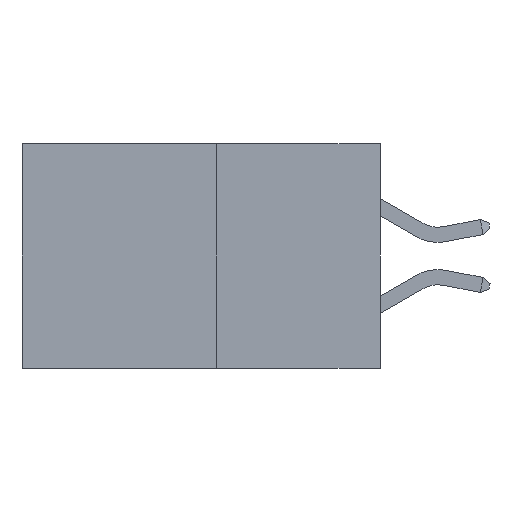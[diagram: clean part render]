
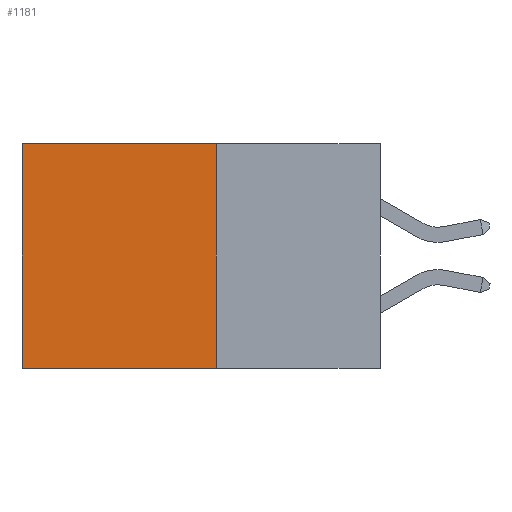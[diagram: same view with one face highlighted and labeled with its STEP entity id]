
A CAD part, left-side view. The second image highlights one B-rep face of the part: STEP entity #1181.
In plain terms, the highlighted planar face has unit normal (-1, 0, 0).
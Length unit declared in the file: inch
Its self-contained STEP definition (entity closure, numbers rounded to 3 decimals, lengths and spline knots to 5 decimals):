
#418 = CARTESIAN_POINT ( 'NONE',  ( 0.277, 0.27, 0. ) ) ;
#1023 = DIRECTION ( 'NONE',  ( 0., 0., -1. ) ) ;
#1181 = ADVANCED_FACE ( 'NONE', ( #3121 ), #8649, .F. ) ;
#1268 = CARTESIAN_POINT ( 'NONE',  ( 0.277, 0.27, -0.37 ) ) ;
#1397 = VERTEX_POINT ( 'NONE', #6415 ) ;
#1732 = DIRECTION ( 'NONE',  ( 0., 1., 0. ) ) ;
#1752 = VECTOR ( 'NONE', #1732, 39.37008 ) ;
#1997 = ORIENTED_EDGE ( 'NONE', *, *, #8250, .F. ) ;
#2171 = VERTEX_POINT ( 'NONE', #4572 ) ;
#2294 = AXIS2_PLACEMENT_3D ( 'NONE', #2335, #6677, #6979 ) ;
#2335 = CARTESIAN_POINT ( 'NONE',  ( 0.277, 0.27, -0.37 ) ) ;
#2494 = ORIENTED_EDGE ( 'NONE', *, *, #2609, .F. ) ;
#2504 = VECTOR ( 'NONE', #9385, 39.37008 ) ;
#2609 = EDGE_CURVE ( 'NONE', #1397, #2171, #6265, .T. ) ;
#2628 = EDGE_CURVE ( 'NONE', #4835, #2171, #8755, .T. ) ;
#2877 = ORIENTED_EDGE ( 'NONE', *, *, #2628, .T. ) ;
#3024 = CARTESIAN_POINT ( 'NONE',  ( 0.277, 0.59, 0. ) ) ;
#3121 = FACE_OUTER_BOUND ( 'NONE', #4414, .T. ) ;
#3892 = VECTOR ( 'NONE', #7174, 39.37008 ) ;
#3923 = EDGE_CURVE ( 'NONE', #6379, #4835, #7024, .T. ) ;
#4414 = EDGE_LOOP ( 'NONE', ( #2877, #2494, #1997, #8170 ) ) ;
#4572 = CARTESIAN_POINT ( 'NONE',  ( 0.277, 0.59, -0.37 ) ) ;
#4835 = VERTEX_POINT ( 'NONE', #3024 ) ;
#5214 = CARTESIAN_POINT ( 'NONE',  ( 0.277, 0.27, 0. ) ) ;
#6265 = LINE ( 'NONE', #8397, #1752 ) ;
#6307 = CARTESIAN_POINT ( 'NONE',  ( 0.277, 0.59, -0.37 ) ) ;
#6379 = VERTEX_POINT ( 'NONE', #418 ) ;
#6415 = CARTESIAN_POINT ( 'NONE',  ( 0.277, 0.27, -0.37 ) ) ;
#6420 = LINE ( 'NONE', #1268, #3892 ) ;
#6677 = DIRECTION ( 'NONE',  ( 1., 0., 0. ) ) ;
#6979 = DIRECTION ( 'NONE',  ( 0., 0., -1. ) ) ;
#7024 = LINE ( 'NONE', #5214, #2504 ) ;
#7174 = DIRECTION ( 'NONE',  ( 0., 0., -1. ) ) ;
#8170 = ORIENTED_EDGE ( 'NONE', *, *, #3923, .T. ) ;
#8250 = EDGE_CURVE ( 'NONE', #6379, #1397, #6420, .T. ) ;
#8397 = CARTESIAN_POINT ( 'NONE',  ( 0.277, 0.27, -0.37 ) ) ;
#8494 = VECTOR ( 'NONE', #1023, 39.37008 ) ;
#8649 = PLANE ( 'NONE',  #2294 ) ;
#8755 = LINE ( 'NONE', #6307, #8494 ) ;
#9385 = DIRECTION ( 'NONE',  ( 0., 1., 0. ) ) ;
